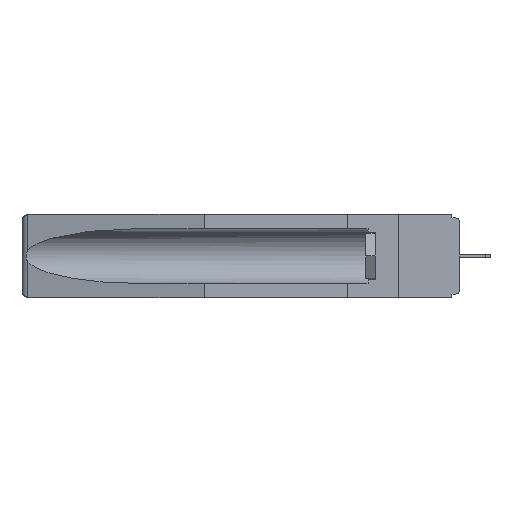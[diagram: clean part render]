
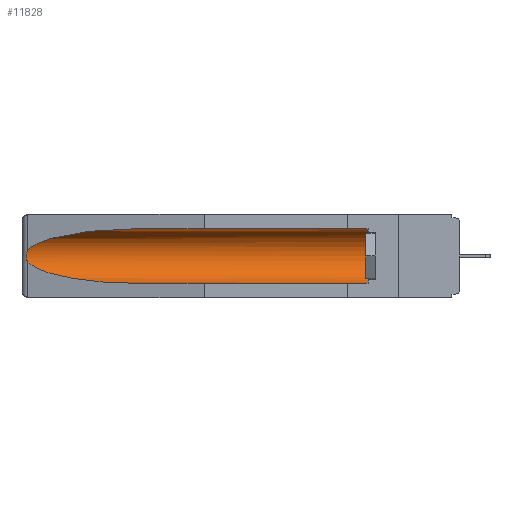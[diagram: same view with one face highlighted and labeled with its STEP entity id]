
A CAD part, left-side view. The second image highlights one B-rep face of the part: STEP entity #11828.
In plain terms, the highlighted cylindrical face has radius 2.857 mm (diameter 5.715 mm), a partial arc.
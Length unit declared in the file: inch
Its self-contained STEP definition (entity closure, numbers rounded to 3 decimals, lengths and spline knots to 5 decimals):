
#42 =( BOUNDED_CURVE ( )  B_SPLINE_CURVE ( 3, ( #7715, #18769, #11233, #11129 ),
 .UNSPECIFIED., .F., .F. ) 
 B_SPLINE_CURVE_WITH_KNOTS ( ( 4, 4 ),
 ( 0.1948, 1.5708 ),
 .UNSPECIFIED. ) 
 CURVE ( )  GEOMETRIC_REPRESENTATION_ITEM ( )  RATIONAL_B_SPLINE_CURVE ( ( 1., 0.848, 0.848, 1. ) ) 
 REPRESENTATION_ITEM ( '' )  );
#452 = CARTESIAN_POINT ( 'NONE',  ( 0.155, 1.07973, -0.059 ) ) ;
#573 = CARTESIAN_POINT ( 'NONE',  ( 0.155, -0.30754, -0.059 ) ) ;
#745 = ORIENTED_EDGE ( 'NONE', *, *, #6305, .T. ) ;
#999 = ORIENTED_EDGE ( 'NONE', *, *, #18555, .T. ) ;
#1117 = CARTESIAN_POINT ( 'NONE',  ( 0.26537, 1.52718, -0.14972 ) ) ;
#1218 = CARTESIAN_POINT ( 'NONE',  ( 0.2673, 1.5327, -0.16383 ) ) ;
#1300 = EDGE_CURVE ( 'NONE', #16383, #17523, #2449, .T. ) ;
#1729 = CARTESIAN_POINT ( 'NONE',  ( 0.155, -0.30754, -0.1715 ) ) ;
#2449 = B_SPLINE_CURVE_WITH_KNOTS ( 'NONE', 3,
 ( #1117, #6070, #2731, #1218, #19533, #3026, #5753, #2924, #8890, #9198 ),
 .UNSPECIFIED., .F., .F.,
 ( 4, 2, 2, 2, 4 ),
 ( 0., 0.00029, 0.00058, 0.00087, 0.00117 ),
 .UNSPECIFIED. ) ;
#2731 = CARTESIAN_POINT ( 'NONE',  ( 0.26654, 1.53092, -0.15636 ) ) ;
#2924 = CARTESIAN_POINT ( 'NONE',  ( 0.26655, 1.53094, -0.18657 ) ) ;
#2966 = CIRCLE ( 'NONE', #16811, 0.1125 ) ;
#3026 = CARTESIAN_POINT ( 'NONE',  ( 0.2675, 1.53308, -0.17534 ) ) ;
#3293 = DIRECTION ( 'NONE',  ( 0., 1., 0. ) ) ;
#4754 = CYLINDRICAL_SURFACE ( 'NONE', #5863, 0.1125 ) ;
#4864 = VERTEX_POINT ( 'NONE', #452 ) ;
#5572 = EDGE_LOOP ( 'NONE', ( #15767, #15623, #6454, #7602, #745, #999 ) ) ;
#5598 = CARTESIAN_POINT ( 'NONE',  ( 0.155, 1.07973, -0.059 ) ) ;
#5753 = CARTESIAN_POINT ( 'NONE',  ( 0.2673, 1.53269, -0.17917 ) ) ;
#5863 = AXIS2_PLACEMENT_3D ( 'NONE', #1729, #10716, #6385 ) ;
#6070 = CARTESIAN_POINT ( 'NONE',  ( 0.26597, 1.52961, -0.15275 ) ) ;
#6305 = EDGE_CURVE ( 'NONE', #7464, #7492, #2966, .T. ) ;
#6385 = DIRECTION ( 'NONE',  ( 0., 0., 1. ) ) ;
#6454 = ORIENTED_EDGE ( 'NONE', *, *, #17688, .T. ) ;
#7267 = LINE ( 'NONE', #573, #10533 ) ;
#7464 = VERTEX_POINT ( 'NONE', #9953 ) ;
#7492 = VERTEX_POINT ( 'NONE', #7614 ) ;
#7602 = ORIENTED_EDGE ( 'NONE', *, *, #8621, .F. ) ;
#7614 = CARTESIAN_POINT ( 'NONE',  ( 0.155, 0.126, -0.059 ) ) ;
#7715 = CARTESIAN_POINT ( 'NONE',  ( 0.26537, 1.52718, -0.19328 ) ) ;
#8157 = CARTESIAN_POINT ( 'NONE',  ( 0.155, -0.30754, -0.284 ) ) ;
#8523 = VECTOR ( 'NONE', #14186, 39.37008 ) ;
#8621 = EDGE_CURVE ( 'NONE', #7464, #18680, #11073, .T. ) ;
#8890 = CARTESIAN_POINT ( 'NONE',  ( 0.26597, 1.5296, -0.19026 ) ) ;
#9198 = CARTESIAN_POINT ( 'NONE',  ( 0.26537, 1.52718, -0.19328 ) ) ;
#9634 = CARTESIAN_POINT ( 'NONE',  ( 0.26537, 1.52718, -0.14972 ) ) ;
#9862 = CARTESIAN_POINT ( 'NONE',  ( 0.25451, 1.48313, -0.09465 ) ) ;
#9953 = CARTESIAN_POINT ( 'NONE',  ( 0.155, 0.126, -0.284 ) ) ;
#10533 = VECTOR ( 'NONE', #3293, 39.37008 ) ;
#10716 = DIRECTION ( 'NONE',  ( 0., 1., 0. ) ) ;
#11073 = LINE ( 'NONE', #8157, #8523 ) ;
#11129 = CARTESIAN_POINT ( 'NONE',  ( 0.155, 1.07973, -0.284 ) ) ;
#11180 = EDGE_CURVE ( 'NONE', #4864, #16383, #13131, .T. ) ;
#11233 = CARTESIAN_POINT ( 'NONE',  ( 0.21114, 1.30732, -0.284 ) ) ;
#11723 = DIRECTION ( 'NONE',  ( 0., -1., 0. ) ) ;
#11736 = CARTESIAN_POINT ( 'NONE',  ( 0.21114, 1.30732, -0.059 ) ) ;
#11828 = ADVANCED_FACE ( 'NONE', ( #12207 ), #4754, .F. ) ;
#11919 = CARTESIAN_POINT ( 'NONE',  ( 0.26537, 1.52718, -0.19328 ) ) ;
#12207 = FACE_OUTER_BOUND ( 'NONE', #5572, .T. ) ;
#13131 =( BOUNDED_CURVE ( )  B_SPLINE_CURVE ( 3, ( #5598, #11736, #9862, #15877 ),
 .UNSPECIFIED., .F., .F. ) 
 B_SPLINE_CURVE_WITH_KNOTS ( ( 4, 4 ),
 ( 4.71239, 6.08839 ),
 .UNSPECIFIED. ) 
 CURVE ( )  GEOMETRIC_REPRESENTATION_ITEM ( )  RATIONAL_B_SPLINE_CURVE ( ( 1., 0.848, 0.848, 1. ) ) 
 REPRESENTATION_ITEM ( '' )  );
#14186 = DIRECTION ( 'NONE',  ( 0., 1., 0. ) ) ;
#14573 = CARTESIAN_POINT ( 'NONE',  ( 0.155, 1.07973, -0.284 ) ) ;
#15623 = ORIENTED_EDGE ( 'NONE', *, *, #1300, .T. ) ;
#15767 = ORIENTED_EDGE ( 'NONE', *, *, #11180, .T. ) ;
#15877 = CARTESIAN_POINT ( 'NONE',  ( 0.26537, 1.52718, -0.14972 ) ) ;
#16373 = CARTESIAN_POINT ( 'NONE',  ( 0.155, 0.126, -0.1715 ) ) ;
#16383 = VERTEX_POINT ( 'NONE', #9634 ) ;
#16811 = AXIS2_PLACEMENT_3D ( 'NONE', #16373, #11723, #19571 ) ;
#17523 = VERTEX_POINT ( 'NONE', #11919 ) ;
#17688 = EDGE_CURVE ( 'NONE', #17523, #18680, #42, .T. ) ;
#18555 = EDGE_CURVE ( 'NONE', #7492, #4864, #7267, .T. ) ;
#18680 = VERTEX_POINT ( 'NONE', #14573 ) ;
#18769 = CARTESIAN_POINT ( 'NONE',  ( 0.25451, 1.48313, -0.24835 ) ) ;
#19533 = CARTESIAN_POINT ( 'NONE',  ( 0.2675, 1.53308, -0.16763 ) ) ;
#19571 = DIRECTION ( 'NONE',  ( 0., 0., 1. ) ) ;
